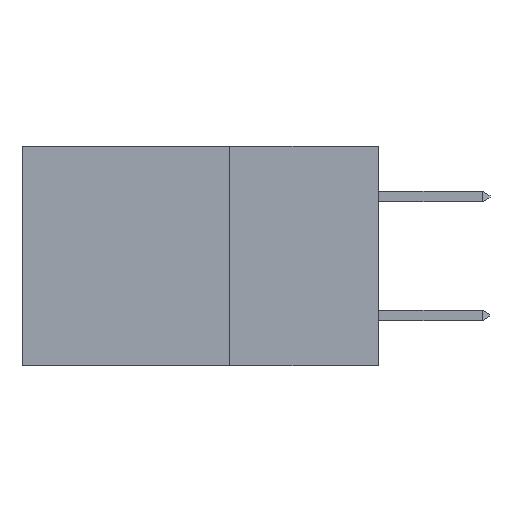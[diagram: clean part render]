
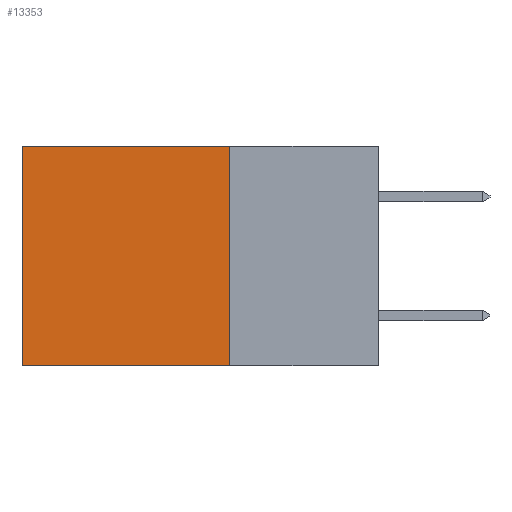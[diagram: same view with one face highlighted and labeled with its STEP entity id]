
A CAD part, left-side view. The second image highlights one B-rep face of the part: STEP entity #13353.
In plain terms, the highlighted planar face has unit normal (-1, 0, 0).
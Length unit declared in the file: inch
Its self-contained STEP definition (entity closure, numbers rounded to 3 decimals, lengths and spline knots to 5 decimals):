
#358 = DIRECTION ( 'NONE',  ( 0., 0., -1. ) ) ;
#380 = DIRECTION ( 'NONE',  ( 0., 1., 0. ) ) ;
#994 = LINE ( 'NONE', #10955, #13310 ) ;
#1224 = EDGE_CURVE ( 'NONE', #3220, #1751, #8574, .T. ) ;
#1610 = CARTESIAN_POINT ( 'NONE',  ( 0.298, 0.6, 0. ) ) ;
#1751 = VERTEX_POINT ( 'NONE', #6850 ) ;
#1798 = DIRECTION ( 'NONE',  ( 0., 0., -1. ) ) ;
#1807 = CARTESIAN_POINT ( 'NONE',  ( 0.298, 0.25, 0. ) ) ;
#1864 = CARTESIAN_POINT ( 'NONE',  ( 0.298, 0.25, -0.37 ) ) ;
#1920 = ORIENTED_EDGE ( 'NONE', *, *, #3219, .F. ) ;
#1980 = VECTOR ( 'NONE', #6734, 39.37008 ) ;
#2438 = VERTEX_POINT ( 'NONE', #12872 ) ;
#3219 = EDGE_CURVE ( 'NONE', #2438, #3220, #13890, .T. ) ;
#3220 = VERTEX_POINT ( 'NONE', #1864 ) ;
#4068 = EDGE_CURVE ( 'NONE', #2438, #13086, #994, .T. ) ;
#4124 = VECTOR ( 'NONE', #1798, 39.37008 ) ;
#4439 = ORIENTED_EDGE ( 'NONE', *, *, #11418, .T. ) ;
#4794 = FACE_OUTER_BOUND ( 'NONE', #5186, .T. ) ;
#5186 = EDGE_LOOP ( 'NONE', ( #4439, #13981, #1920, #9746 ) ) ;
#6734 = DIRECTION ( 'NONE',  ( 0., 1., 0. ) ) ;
#6850 = CARTESIAN_POINT ( 'NONE',  ( 0.298, 0.6, -0.37 ) ) ;
#7813 = DIRECTION ( 'NONE',  ( 1., 0., 0. ) ) ;
#8036 = LINE ( 'NONE', #8790, #14103 ) ;
#8574 = LINE ( 'NONE', #9336, #1980 ) ;
#8790 = CARTESIAN_POINT ( 'NONE',  ( 0.298, 0.6, 0. ) ) ;
#9336 = CARTESIAN_POINT ( 'NONE',  ( 0.298, 0.25, -0.37 ) ) ;
#9746 = ORIENTED_EDGE ( 'NONE', *, *, #4068, .T. ) ;
#9957 = DIRECTION ( 'NONE',  ( 0., 0., -1. ) ) ;
#10026 = AXIS2_PLACEMENT_3D ( 'NONE', #11323, #7813, #358 ) ;
#10955 = CARTESIAN_POINT ( 'NONE',  ( 0.298, 0.25, 0. ) ) ;
#11323 = CARTESIAN_POINT ( 'NONE',  ( 0.298, 0.25, 0. ) ) ;
#11418 = EDGE_CURVE ( 'NONE', #13086, #1751, #8036, .T. ) ;
#12667 = PLANE ( 'NONE',  #10026 ) ;
#12872 = CARTESIAN_POINT ( 'NONE',  ( 0.298, 0.25, 0. ) ) ;
#13086 = VERTEX_POINT ( 'NONE', #1610 ) ;
#13310 = VECTOR ( 'NONE', #380, 39.37008 ) ;
#13353 = ADVANCED_FACE ( 'NONE', ( #4794 ), #12667, .F. ) ;
#13890 = LINE ( 'NONE', #1807, #4124 ) ;
#13981 = ORIENTED_EDGE ( 'NONE', *, *, #1224, .F. ) ;
#14103 = VECTOR ( 'NONE', #9957, 39.37008 ) ;
